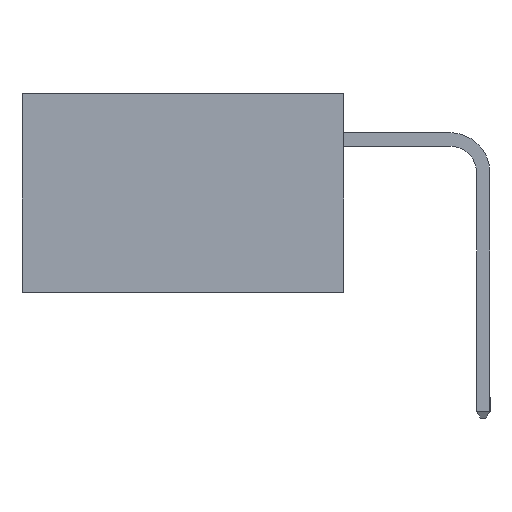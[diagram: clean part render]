
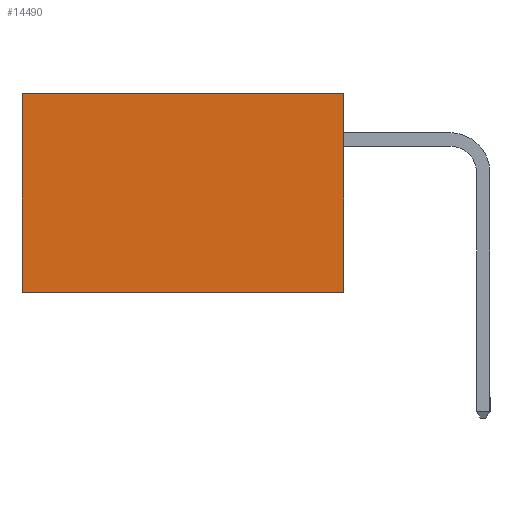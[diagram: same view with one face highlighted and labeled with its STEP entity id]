
A CAD part, left-side view. The second image highlights one B-rep face of the part: STEP entity #14490.
In plain terms, the highlighted planar face has unit normal (-1, 0, 0).
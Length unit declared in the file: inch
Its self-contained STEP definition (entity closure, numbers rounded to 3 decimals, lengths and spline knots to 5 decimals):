
#686 = CARTESIAN_POINT ( 'NONE',  ( 0.2615, 0.6, -0.37 ) ) ;
#1219 = EDGE_CURVE ( 'NONE', #7641, #12698, #15556, .T. ) ;
#1596 = DIRECTION ( 'NONE',  ( 0., 0., -1. ) ) ;
#1832 = VECTOR ( 'NONE', #6647, 39.37008 ) ;
#2338 = LINE ( 'NONE', #3379, #16401 ) ;
#3077 = ORIENTED_EDGE ( 'NONE', *, *, #1219, .T. ) ;
#3247 = DIRECTION ( 'NONE',  ( 0., 0., -1. ) ) ;
#3379 = CARTESIAN_POINT ( 'NONE',  ( 0.2615, 0., -0.37 ) ) ;
#3601 = VECTOR ( 'NONE', #16816, 39.37008 ) ;
#4639 = EDGE_CURVE ( 'NONE', #17940, #16947, #2338, .T. ) ;
#4806 = ORIENTED_EDGE ( 'NONE', *, *, #17823, .T. ) ;
#5006 = CARTESIAN_POINT ( 'NONE',  ( 0.2615, 0., -0.37 ) ) ;
#5335 = EDGE_LOOP ( 'NONE', ( #3077, #15020, #17980, #4806 ) ) ;
#5398 = CARTESIAN_POINT ( 'NONE',  ( 0.2615, 0.6, -0.37 ) ) ;
#6647 = DIRECTION ( 'NONE',  ( 0., 0., -1. ) ) ;
#7641 = VERTEX_POINT ( 'NONE', #20236 ) ;
#7788 = CARTESIAN_POINT ( 'NONE',  ( 0.2615, 0., -0.37 ) ) ;
#8608 = FACE_OUTER_BOUND ( 'NONE', #5335, .T. ) ;
#10358 = PLANE ( 'NONE',  #22592 ) ;
#12134 = DIRECTION ( 'NONE',  ( 1., 0., 0. ) ) ;
#12698 = VERTEX_POINT ( 'NONE', #686 ) ;
#12935 = LINE ( 'NONE', #15052, #3601 ) ;
#14082 = EDGE_CURVE ( 'NONE', #16947, #12698, #19834, .T. ) ;
#14490 = ADVANCED_FACE ( 'NONE', ( #8608 ), #10358, .F. ) ;
#15020 = ORIENTED_EDGE ( 'NONE', *, *, #14082, .F. ) ;
#15052 = CARTESIAN_POINT ( 'NONE',  ( 0.2615, 0., 0. ) ) ;
#15556 = LINE ( 'NONE', #5398, #1832 ) ;
#16240 = VECTOR ( 'NONE', #16809, 39.37008 ) ;
#16401 = VECTOR ( 'NONE', #3247, 39.37008 ) ;
#16809 = DIRECTION ( 'NONE',  ( 0., 1., 0. ) ) ;
#16816 = DIRECTION ( 'NONE',  ( 0., 1., 0. ) ) ;
#16947 = VERTEX_POINT ( 'NONE', #7788 ) ;
#17823 = EDGE_CURVE ( 'NONE', #17940, #7641, #12935, .T. ) ;
#17940 = VERTEX_POINT ( 'NONE', #18917 ) ;
#17980 = ORIENTED_EDGE ( 'NONE', *, *, #4639, .F. ) ;
#18917 = CARTESIAN_POINT ( 'NONE',  ( 0.2615, 0., 0. ) ) ;
#19834 = LINE ( 'NONE', #20272, #16240 ) ;
#20236 = CARTESIAN_POINT ( 'NONE',  ( 0.2615, 0.6, 0. ) ) ;
#20272 = CARTESIAN_POINT ( 'NONE',  ( 0.2615, 0., -0.37 ) ) ;
#22592 = AXIS2_PLACEMENT_3D ( 'NONE', #5006, #12134, #1596 ) ;
